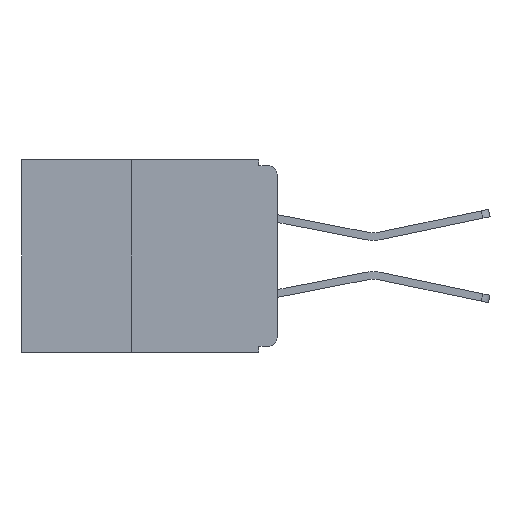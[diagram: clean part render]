
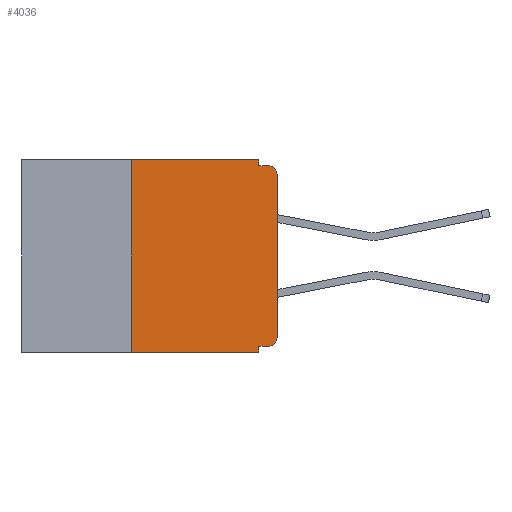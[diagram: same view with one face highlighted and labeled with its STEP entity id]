
A CAD part, left-side view. The second image highlights one B-rep face of the part: STEP entity #4036.
In plain terms, the highlighted planar face has unit normal (-1, 0, 0).
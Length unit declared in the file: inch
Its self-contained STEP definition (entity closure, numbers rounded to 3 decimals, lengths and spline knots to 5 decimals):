
#468 = DIRECTION ( 'NONE',  ( 0., 0., -1. ) ) ;
#652 = EDGE_CURVE ( 'NONE', #9475, #11913, #2695, .T. ) ;
#1029 = LINE ( 'NONE', #18654, #14022 ) ;
#1367 = CARTESIAN_POINT ( 'NONE',  ( 0., 0.437, -0.33 ) ) ;
#1610 = VECTOR ( 'NONE', #9546, 39.37008 ) ;
#1811 = CARTESIAN_POINT ( 'NONE',  ( 0., 0.015, -0.025 ) ) ;
#2695 = LINE ( 'NONE', #17525, #1610 ) ;
#2833 = ORIENTED_EDGE ( 'NONE', *, *, #10617, .F. ) ;
#3059 = VECTOR ( 'NONE', #21219, 39.37008 ) ;
#3078 = DIRECTION ( 'NONE',  ( 0., -1., 0. ) ) ;
#3096 = CIRCLE ( 'NONE', #16818, 0.015 ) ;
#3240 = EDGE_CURVE ( 'NONE', #5945, #19435, #9244, .T. ) ;
#3545 = DIRECTION ( 'NONE',  ( 0., 0., -1. ) ) ;
#3832 = CARTESIAN_POINT ( 'NONE',  ( 0., 0.437, 0. ) ) ;
#3833 = ORIENTED_EDGE ( 'NONE', *, *, #3240, .F. ) ;
#3843 = AXIS2_PLACEMENT_3D ( 'NONE', #1811, #13655, #3545 ) ;
#3856 = VECTOR ( 'NONE', #20023, 39.37008 ) ;
#4036 = ADVANCED_FACE ( 'NONE', ( #18192 ), #15654, .F. ) ;
#5614 = CARTESIAN_POINT ( 'NONE',  ( 0., 0., 0. ) ) ;
#5913 = ORIENTED_EDGE ( 'NONE', *, *, #12971, .T. ) ;
#5945 = VERTEX_POINT ( 'NONE', #20784 ) ;
#5997 = DIRECTION ( 'NONE',  ( 0., 0., -1. ) ) ;
#6377 = EDGE_CURVE ( 'NONE', #16038, #17587, #11064, .T. ) ;
#6770 = EDGE_CURVE ( 'NONE', #12030, #15070, #13170, .T. ) ;
#6835 = CARTESIAN_POINT ( 'NONE',  ( 0., 0.015, -0.32 ) ) ;
#7100 = CARTESIAN_POINT ( 'NONE',  ( 0., 0.015, -0.305 ) ) ;
#7101 = VECTOR ( 'NONE', #5997, 39.37008 ) ;
#7324 = DIRECTION ( 'NONE',  ( 0., 0., 1. ) ) ;
#7883 = CARTESIAN_POINT ( 'NONE',  ( 0., 0., -0.305 ) ) ;
#8505 = DIRECTION ( 'NONE',  ( 0., -1., 0. ) ) ;
#8510 = EDGE_CURVE ( 'NONE', #15070, #18513, #9421, .T. ) ;
#8551 = CARTESIAN_POINT ( 'NONE',  ( 0., 0., -0.025 ) ) ;
#8800 = DIRECTION ( 'NONE',  ( 0., 0., -1. ) ) ;
#8914 = CARTESIAN_POINT ( 'NONE',  ( 0., 0.25, 0. ) ) ;
#9244 = LINE ( 'NONE', #17054, #12138 ) ;
#9421 = CIRCLE ( 'NONE', #3843, 0.015 ) ;
#9475 = VERTEX_POINT ( 'NONE', #12310 ) ;
#9546 = DIRECTION ( 'NONE',  ( 0., 0., 1. ) ) ;
#10067 = ORIENTED_EDGE ( 'NONE', *, *, #6377, .F. ) ;
#10492 = EDGE_CURVE ( 'NONE', #9475, #17587, #21232, .T. ) ;
#10617 = EDGE_CURVE ( 'NONE', #11913, #5945, #1029, .T. ) ;
#10641 = DIRECTION ( 'NONE',  ( 1., 0., 0. ) ) ;
#10865 = ORIENTED_EDGE ( 'NONE', *, *, #10492, .T. ) ;
#10923 = CARTESIAN_POINT ( 'NONE',  ( 0., 0.031, -0.33 ) ) ;
#11064 = LINE ( 'NONE', #17842, #7101 ) ;
#11913 = VERTEX_POINT ( 'NONE', #8914 ) ;
#12030 = VERTEX_POINT ( 'NONE', #7883 ) ;
#12138 = VECTOR ( 'NONE', #20393, 39.37008 ) ;
#12143 = ORIENTED_EDGE ( 'NONE', *, *, #6770, .T. ) ;
#12191 = VECTOR ( 'NONE', #3078, 39.37008 ) ;
#12310 = CARTESIAN_POINT ( 'NONE',  ( 0., 0.25, -0.33 ) ) ;
#12971 = EDGE_CURVE ( 'NONE', #14183, #12030, #3096, .T. ) ;
#13170 = LINE ( 'NONE', #5614, #17145 ) ;
#13383 = CARTESIAN_POINT ( 'NONE',  ( 0., 0.015, -0.01 ) ) ;
#13655 = DIRECTION ( 'NONE',  ( -1., 0., 0. ) ) ;
#13842 = EDGE_CURVE ( 'NONE', #19435, #18513, #16587, .T. ) ;
#14022 = VECTOR ( 'NONE', #8505, 39.37008 ) ;
#14034 = EDGE_CURVE ( 'NONE', #14183, #16038, #17902, .T. ) ;
#14183 = VERTEX_POINT ( 'NONE', #6835 ) ;
#14862 = CARTESIAN_POINT ( 'NONE',  ( 0., 0., -0.32 ) ) ;
#15070 = VERTEX_POINT ( 'NONE', #8551 ) ;
#15324 = ORIENTED_EDGE ( 'NONE', *, *, #652, .F. ) ;
#15654 = PLANE ( 'NONE',  #19692 ) ;
#15777 = CARTESIAN_POINT ( 'NONE',  ( 0., 0.031, -0.01 ) ) ;
#16038 = VERTEX_POINT ( 'NONE', #16097 ) ;
#16097 = CARTESIAN_POINT ( 'NONE',  ( 0., 0.031, -0.32 ) ) ;
#16587 = LINE ( 'NONE', #19510, #3059 ) ;
#16818 = AXIS2_PLACEMENT_3D ( 'NONE', #7100, #18940, #8800 ) ;
#17054 = CARTESIAN_POINT ( 'NONE',  ( 0., 0.031, 0. ) ) ;
#17145 = VECTOR ( 'NONE', #7324, 39.37008 ) ;
#17525 = CARTESIAN_POINT ( 'NONE',  ( 0., 0.25, -0.33 ) ) ;
#17587 = VERTEX_POINT ( 'NONE', #10923 ) ;
#17842 = CARTESIAN_POINT ( 'NONE',  ( 0., 0.031, -0.33 ) ) ;
#17902 = LINE ( 'NONE', #14862, #3856 ) ;
#18192 = FACE_OUTER_BOUND ( 'NONE', #20348, .T. ) ;
#18513 = VERTEX_POINT ( 'NONE', #13383 ) ;
#18654 = CARTESIAN_POINT ( 'NONE',  ( 0., 0.437, 0. ) ) ;
#18807 = ORIENTED_EDGE ( 'NONE', *, *, #14034, .F. ) ;
#18940 = DIRECTION ( 'NONE',  ( -1., 0., 0. ) ) ;
#19435 = VERTEX_POINT ( 'NONE', #15777 ) ;
#19510 = CARTESIAN_POINT ( 'NONE',  ( 0., 0., -0.01 ) ) ;
#19692 = AXIS2_PLACEMENT_3D ( 'NONE', #3832, #10641, #468 ) ;
#20023 = DIRECTION ( 'NONE',  ( 0., 1., 0. ) ) ;
#20348 = EDGE_LOOP ( 'NONE', ( #12143, #20704, #20802, #3833, #2833, #15324, #10865, #10067, #18807, #5913 ) ) ;
#20393 = DIRECTION ( 'NONE',  ( 0., 0., -1. ) ) ;
#20704 = ORIENTED_EDGE ( 'NONE', *, *, #8510, .T. ) ;
#20784 = CARTESIAN_POINT ( 'NONE',  ( 0., 0.031, 0. ) ) ;
#20802 = ORIENTED_EDGE ( 'NONE', *, *, #13842, .F. ) ;
#21219 = DIRECTION ( 'NONE',  ( 0., -1., 0. ) ) ;
#21232 = LINE ( 'NONE', #1367, #12191 ) ;
